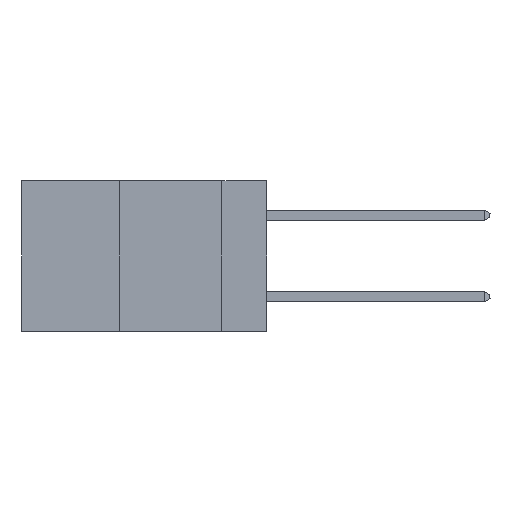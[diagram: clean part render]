
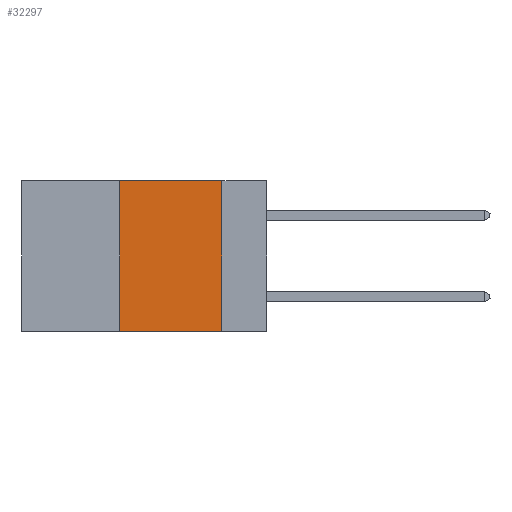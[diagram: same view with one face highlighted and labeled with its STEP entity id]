
A CAD part, left-side view. The second image highlights one B-rep face of the part: STEP entity #32297.
In plain terms, the highlighted planar face has unit normal (-1, 0, 0).
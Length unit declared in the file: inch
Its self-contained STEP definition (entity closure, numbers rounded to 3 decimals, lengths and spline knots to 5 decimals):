
#243 = EDGE_CURVE ( 'NONE', #18194, #14067, #20645, .T. ) ;
#728 = EDGE_CURVE ( 'NONE', #14067, #20012, #8971, .T. ) ;
#1911 = DIRECTION ( 'NONE',  ( 1., 0., 0. ) ) ;
#2938 = DIRECTION ( 'NONE',  ( 0., -1., 0. ) ) ;
#6127 = CARTESIAN_POINT ( 'NONE',  ( 0., 0.36, 0. ) ) ;
#6440 = CARTESIAN_POINT ( 'NONE',  ( 0., 0.11, 0. ) ) ;
#6685 = VECTOR ( 'NONE', #33264, 39.37008 ) ;
#7288 = ORIENTED_EDGE ( 'NONE', *, *, #728, .F. ) ;
#8971 = LINE ( 'NONE', #6440, #26596 ) ;
#9119 = CARTESIAN_POINT ( 'NONE',  ( 0., 0.6, 0. ) ) ;
#9472 = ORIENTED_EDGE ( 'NONE', *, *, #12760, .F. ) ;
#12760 = EDGE_CURVE ( 'NONE', #27421, #18194, #29711, .T. ) ;
#12840 = CARTESIAN_POINT ( 'NONE',  ( 0., 0.11, 0. ) ) ;
#13710 = PLANE ( 'NONE',  #31999 ) ;
#14067 = VERTEX_POINT ( 'NONE', #12840 ) ;
#14828 = EDGE_LOOP ( 'NONE', ( #7288, #17124, #9472, #25745 ) ) ;
#17124 = ORIENTED_EDGE ( 'NONE', *, *, #243, .F. ) ;
#17776 = DIRECTION ( 'NONE',  ( 0., 0., 1. ) ) ;
#18194 = VERTEX_POINT ( 'NONE', #6127 ) ;
#20012 = VERTEX_POINT ( 'NONE', #31384 ) ;
#20645 = LINE ( 'NONE', #9119, #6685 ) ;
#25622 = VECTOR ( 'NONE', #2938, 39.37008 ) ;
#25745 = ORIENTED_EDGE ( 'NONE', *, *, #26656, .T. ) ;
#26596 = VECTOR ( 'NONE', #35525, 39.37008 ) ;
#26656 = EDGE_CURVE ( 'NONE', #27421, #20012, #38035, .T. ) ;
#27421 = VERTEX_POINT ( 'NONE', #27814 ) ;
#27814 = CARTESIAN_POINT ( 'NONE',  ( 0., 0.36, -0.37 ) ) ;
#29711 = LINE ( 'NONE', #35425, #37519 ) ;
#31384 = CARTESIAN_POINT ( 'NONE',  ( 0., 0.11, -0.37 ) ) ;
#31999 = AXIS2_PLACEMENT_3D ( 'NONE', #37372, #1911, #37486 ) ;
#32297 = ADVANCED_FACE ( 'NONE', ( #34831 ), #13710, .F. ) ;
#33264 = DIRECTION ( 'NONE',  ( 0., -1., 0. ) ) ;
#34831 = FACE_OUTER_BOUND ( 'NONE', #14828, .T. ) ;
#35271 = CARTESIAN_POINT ( 'NONE',  ( 0., 0.6, -0.37 ) ) ;
#35425 = CARTESIAN_POINT ( 'NONE',  ( 0., 0.36, 0. ) ) ;
#35525 = DIRECTION ( 'NONE',  ( 0., 0., -1. ) ) ;
#37372 = CARTESIAN_POINT ( 'NONE',  ( 0., 0.6, 0. ) ) ;
#37486 = DIRECTION ( 'NONE',  ( 0., 0., -1. ) ) ;
#37519 = VECTOR ( 'NONE', #17776, 39.37008 ) ;
#38035 = LINE ( 'NONE', #35271, #25622 ) ;
